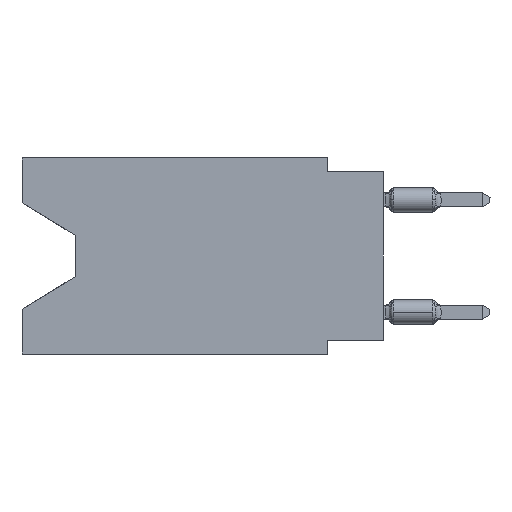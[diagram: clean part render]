
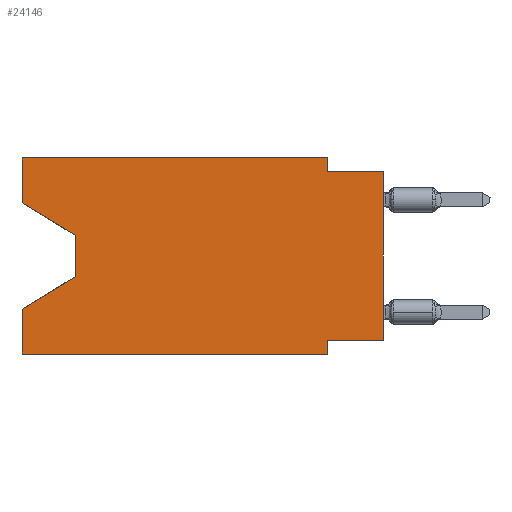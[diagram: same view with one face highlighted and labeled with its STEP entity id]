
A CAD part, left-side view. The second image highlights one B-rep face of the part: STEP entity #24146.
In plain terms, the highlighted planar face has unit normal (-1, 0, 0).
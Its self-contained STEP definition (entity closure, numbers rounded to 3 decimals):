
#69 = ORIENTED_EDGE ( 'NONE', *, *, #25765, .T. ) ;
#374 = LINE ( 'NONE', #16449, #6104 ) ;
#725 = DIRECTION ( 'NONE',  ( 1., 0., 0. ) ) ;
#1069 = VECTOR ( 'NONE', #11659, 1000. ) ;
#1210 = CARTESIAN_POINT ( 'NONE',  ( 0., 16.383, -8.89 ) ) ;
#1842 = CARTESIAN_POINT ( 'NONE',  ( 0., 0., -0.635 ) ) ;
#1986 = CARTESIAN_POINT ( 'NONE',  ( 0., 16.383, 0. ) ) ;
#2528 = ORIENTED_EDGE ( 'NONE', *, *, #11260, .T. ) ;
#2903 = ORIENTED_EDGE ( 'NONE', *, *, #9132, .T. ) ;
#2914 = VERTEX_POINT ( 'NONE', #15134 ) ;
#2983 = LINE ( 'NONE', #8733, #3098 ) ;
#3098 = VECTOR ( 'NONE', #24721, 1000. ) ;
#3485 = CARTESIAN_POINT ( 'NONE',  ( 0., 16.383, 0. ) ) ;
#3497 = VERTEX_POINT ( 'NONE', #14129 ) ;
#3589 = ORIENTED_EDGE ( 'NONE', *, *, #11788, .F. ) ;
#3611 = VERTEX_POINT ( 'NONE', #8889 ) ;
#3817 = ORIENTED_EDGE ( 'NONE', *, *, #10203, .T. ) ;
#3838 = LINE ( 'NONE', #11815, #6693 ) ;
#3953 = CARTESIAN_POINT ( 'NONE',  ( 0., 0., 0. ) ) ;
#4816 = ORIENTED_EDGE ( 'NONE', *, *, #9854, .F. ) ;
#5021 = CARTESIAN_POINT ( 'NONE',  ( 0., 16.383, 0. ) ) ;
#6104 = VECTOR ( 'NONE', #6240, 1000. ) ;
#6240 = DIRECTION ( 'NONE',  ( 0., 0., -1. ) ) ;
#6693 = VECTOR ( 'NONE', #19775, 1000. ) ;
#6975 = DIRECTION ( 'NONE',  ( 0., 0., -1. ) ) ;
#6979 = CARTESIAN_POINT ( 'NONE',  ( 0., 0., -8.255 ) ) ;
#7115 = DIRECTION ( 'NONE',  ( 0., 0.855, -0.519 ) ) ;
#7436 = VECTOR ( 'NONE', #10746, 1000. ) ;
#7473 = LINE ( 'NONE', #13753, #1069 ) ;
#7626 = VECTOR ( 'NONE', #13747, 1000. ) ;
#7864 = DIRECTION ( 'NONE',  ( 0., 0., 1. ) ) ;
#7979 = CARTESIAN_POINT ( 'NONE',  ( 0., 13.97, -3.505 ) ) ;
#8616 = CARTESIAN_POINT ( 'NONE',  ( 0., 2.54, -8.89 ) ) ;
#8642 = VERTEX_POINT ( 'NONE', #19143 ) ;
#8733 = CARTESIAN_POINT ( 'NONE',  ( 0., 16.383, 0. ) ) ;
#8889 = CARTESIAN_POINT ( 'NONE',  ( 0., 2.54, -8.255 ) ) ;
#9039 = CARTESIAN_POINT ( 'NONE',  ( 0., 16.383, -2.038 ) ) ;
#9132 = EDGE_CURVE ( 'NONE', #23881, #9553, #25682, .T. ) ;
#9236 = LINE ( 'NONE', #3485, #24585 ) ;
#9553 = VERTEX_POINT ( 'NONE', #25651 ) ;
#9854 = EDGE_CURVE ( 'NONE', #2914, #11629, #2983, .T. ) ;
#9859 = ORIENTED_EDGE ( 'NONE', *, *, #16259, .F. ) ;
#10199 = ORIENTED_EDGE ( 'NONE', *, *, #24992, .F. ) ;
#10203 = EDGE_CURVE ( 'NONE', #2914, #24458, #21218, .T. ) ;
#10498 = LINE ( 'NONE', #1986, #11787 ) ;
#10702 = ORIENTED_EDGE ( 'NONE', *, *, #12046, .F. ) ;
#10746 = DIRECTION ( 'NONE',  ( 0., -0.855, -0.519 ) ) ;
#10963 = ORIENTED_EDGE ( 'NONE', *, *, #21964, .F. ) ;
#11022 = VERTEX_POINT ( 'NONE', #15894 ) ;
#11260 = EDGE_CURVE ( 'NONE', #9553, #11629, #15228, .T. ) ;
#11629 = VERTEX_POINT ( 'NONE', #13461 ) ;
#11659 = DIRECTION ( 'NONE',  ( 0., 0., -1. ) ) ;
#11755 = AXIS2_PLACEMENT_3D ( 'NONE', #5021, #725, #6975 ) ;
#11787 = VECTOR ( 'NONE', #14031, 1000. ) ;
#11788 = EDGE_CURVE ( 'NONE', #3611, #24458, #374, .T. ) ;
#11815 = CARTESIAN_POINT ( 'NONE',  ( 0., 0., -8.255 ) ) ;
#12046 = EDGE_CURVE ( 'NONE', #8642, #16330, #12524, .T. ) ;
#12524 = LINE ( 'NONE', #20505, #22434 ) ;
#12886 = VECTOR ( 'NONE', #7115, 1000. ) ;
#13461 = CARTESIAN_POINT ( 'NONE',  ( 0., 16.383, -6.852 ) ) ;
#13747 = DIRECTION ( 'NONE',  ( 0., 0., -1. ) ) ;
#13753 = CARTESIAN_POINT ( 'NONE',  ( 0., 2.54, 0. ) ) ;
#13938 = EDGE_CURVE ( 'NONE', #25373, #3611, #3838, .T. ) ;
#14031 = DIRECTION ( 'NONE',  ( 0., 0., 1. ) ) ;
#14129 = CARTESIAN_POINT ( 'NONE',  ( 0., 16.383, -2.038 ) ) ;
#14713 = PLANE ( 'NONE',  #11755 ) ;
#14946 = DIRECTION ( 'NONE',  ( 0., -1., 0. ) ) ;
#14995 = DIRECTION ( 'NONE',  ( 0., -1., 0. ) ) ;
#15134 = CARTESIAN_POINT ( 'NONE',  ( 0., 16.383, -8.89 ) ) ;
#15228 = LINE ( 'NONE', #23211, #12886 ) ;
#15793 = ORIENTED_EDGE ( 'NONE', *, *, #13938, .F. ) ;
#15894 = CARTESIAN_POINT ( 'NONE',  ( 0., 16.383, 0. ) ) ;
#16259 = EDGE_CURVE ( 'NONE', #24093, #8642, #7473, .T. ) ;
#16330 = VERTEX_POINT ( 'NONE', #1842 ) ;
#16449 = CARTESIAN_POINT ( 'NONE',  ( 0., 2.54, -8.89 ) ) ;
#18234 = CARTESIAN_POINT ( 'NONE',  ( 0., 2.54, 0. ) ) ;
#18317 = VECTOR ( 'NONE', #7864, 1000. ) ;
#19004 = FACE_OUTER_BOUND ( 'NONE', #23000, .T. ) ;
#19143 = CARTESIAN_POINT ( 'NONE',  ( 0., 2.54, -0.635 ) ) ;
#19775 = DIRECTION ( 'NONE',  ( 0., 1., 0. ) ) ;
#19927 = CARTESIAN_POINT ( 'NONE',  ( 0., 13.97, -3.505 ) ) ;
#20505 = CARTESIAN_POINT ( 'NONE',  ( 0., 0., -0.635 ) ) ;
#21150 = ORIENTED_EDGE ( 'NONE', *, *, #25556, .T. ) ;
#21218 = LINE ( 'NONE', #1210, #24010 ) ;
#21964 = EDGE_CURVE ( 'NONE', #3497, #11022, #10498, .T. ) ;
#22434 = VECTOR ( 'NONE', #25483, 1000. ) ;
#22911 = LINE ( 'NONE', #9039, #7436 ) ;
#23000 = EDGE_LOOP ( 'NONE', ( #69, #2903, #2528, #4816, #3817, #3589, #15793, #21150, #10702, #9859, #10199, #10963 ) ) ;
#23211 = CARTESIAN_POINT ( 'NONE',  ( 0., 13.97, -5.385 ) ) ;
#23881 = VERTEX_POINT ( 'NONE', #19927 ) ;
#24010 = VECTOR ( 'NONE', #14946, 1000. ) ;
#24093 = VERTEX_POINT ( 'NONE', #18234 ) ;
#24146 = ADVANCED_FACE ( 'NONE', ( #19004 ), #14713, .F. ) ;
#24458 = VERTEX_POINT ( 'NONE', #8616 ) ;
#24585 = VECTOR ( 'NONE', #14995, 1000. ) ;
#24721 = DIRECTION ( 'NONE',  ( 0., 0., 1. ) ) ;
#24992 = EDGE_CURVE ( 'NONE', #11022, #24093, #9236, .T. ) ;
#25373 = VERTEX_POINT ( 'NONE', #6979 ) ;
#25483 = DIRECTION ( 'NONE',  ( 0., -1., 0. ) ) ;
#25556 = EDGE_CURVE ( 'NONE', #25373, #16330, #25578, .T. ) ;
#25578 = LINE ( 'NONE', #3953, #18317 ) ;
#25651 = CARTESIAN_POINT ( 'NONE',  ( 0., 13.97, -5.385 ) ) ;
#25682 = LINE ( 'NONE', #7979, #7626 ) ;
#25765 = EDGE_CURVE ( 'NONE', #3497, #23881, #22911, .T. ) ;
